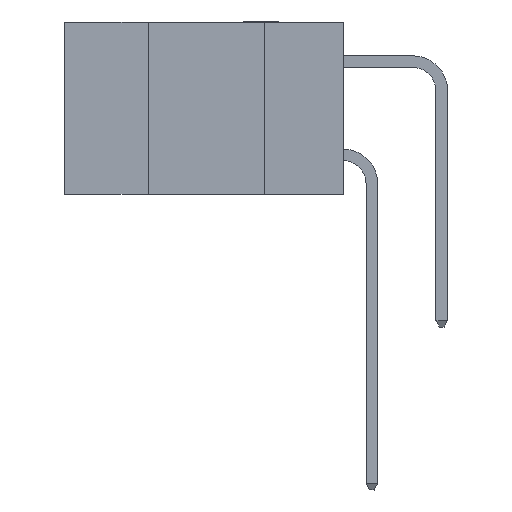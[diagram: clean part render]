
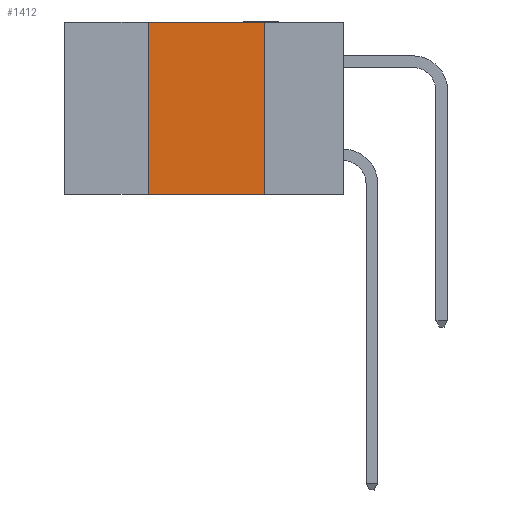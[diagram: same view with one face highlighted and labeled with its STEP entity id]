
A CAD part, left-side view. The second image highlights one B-rep face of the part: STEP entity #1412.
In plain terms, the highlighted planar face has unit normal (-1, 0, 0).
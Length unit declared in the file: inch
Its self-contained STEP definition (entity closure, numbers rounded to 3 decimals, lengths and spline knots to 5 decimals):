
#609 = CARTESIAN_POINT ( 'NONE',  ( 0., 0.17, -0.37 ) ) ;
#1412 = ADVANCED_FACE ( 'NONE', ( #6725 ), #10441, .F. ) ;
#2185 = VECTOR ( 'NONE', #15870, 39.37008 ) ;
#2652 = EDGE_CURVE ( 'NONE', #10299, #9624, #3890, .T. ) ;
#3723 = VERTEX_POINT ( 'NONE', #609 ) ;
#3890 = LINE ( 'NONE', #6226, #13579 ) ;
#4027 = DIRECTION ( 'NONE',  ( 0., 0., -1. ) ) ;
#4598 = EDGE_CURVE ( 'NONE', #9702, #3723, #12353, .T. ) ;
#4640 = CARTESIAN_POINT ( 'NONE',  ( 0., 0.42, 0. ) ) ;
#4995 = EDGE_CURVE ( 'NONE', #9624, #3723, #14105, .T. ) ;
#5221 = VECTOR ( 'NONE', #14058, 39.37008 ) ;
#5414 = AXIS2_PLACEMENT_3D ( 'NONE', #15299, #11592, #4027 ) ;
#6226 = CARTESIAN_POINT ( 'NONE',  ( 0., 0.6, 0. ) ) ;
#6725 = FACE_OUTER_BOUND ( 'NONE', #13208, .T. ) ;
#6833 = CARTESIAN_POINT ( 'NONE',  ( 0., 0.42, -0.37 ) ) ;
#7377 = CARTESIAN_POINT ( 'NONE',  ( 0., 0.6, -0.37 ) ) ;
#8947 = DIRECTION ( 'NONE',  ( 0., -1., 0. ) ) ;
#9010 = ORIENTED_EDGE ( 'NONE', *, *, #4598, .T. ) ;
#9624 = VERTEX_POINT ( 'NONE', #11499 ) ;
#9702 = VERTEX_POINT ( 'NONE', #6833 ) ;
#9814 = VECTOR ( 'NONE', #9821, 39.37008 ) ;
#9821 = DIRECTION ( 'NONE',  ( 0., -1., 0. ) ) ;
#10299 = VERTEX_POINT ( 'NONE', #14591 ) ;
#10441 = PLANE ( 'NONE',  #5414 ) ;
#11499 = CARTESIAN_POINT ( 'NONE',  ( 0., 0.17, 0. ) ) ;
#11592 = DIRECTION ( 'NONE',  ( 1., 0., 0. ) ) ;
#12353 = LINE ( 'NONE', #7377, #9814 ) ;
#13208 = EDGE_LOOP ( 'NONE', ( #16269, #13855, #15220, #9010 ) ) ;
#13579 = VECTOR ( 'NONE', #8947, 39.37008 ) ;
#13855 = ORIENTED_EDGE ( 'NONE', *, *, #2652, .F. ) ;
#13893 = CARTESIAN_POINT ( 'NONE',  ( 0., 0.17, 0. ) ) ;
#14058 = DIRECTION ( 'NONE',  ( 0., 0., -1. ) ) ;
#14105 = LINE ( 'NONE', #13893, #5221 ) ;
#14591 = CARTESIAN_POINT ( 'NONE',  ( 0., 0.42, 0. ) ) ;
#14804 = EDGE_CURVE ( 'NONE', #9702, #10299, #14989, .T. ) ;
#14989 = LINE ( 'NONE', #4640, #2185 ) ;
#15220 = ORIENTED_EDGE ( 'NONE', *, *, #14804, .F. ) ;
#15299 = CARTESIAN_POINT ( 'NONE',  ( 0., 0.6, 0. ) ) ;
#15870 = DIRECTION ( 'NONE',  ( 0., 0., 1. ) ) ;
#16269 = ORIENTED_EDGE ( 'NONE', *, *, #4995, .F. ) ;
